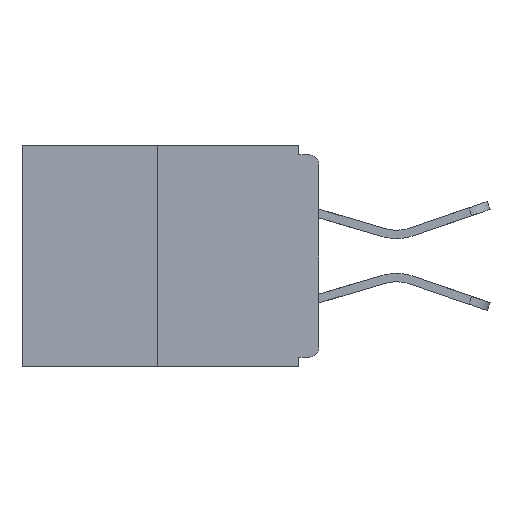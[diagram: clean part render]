
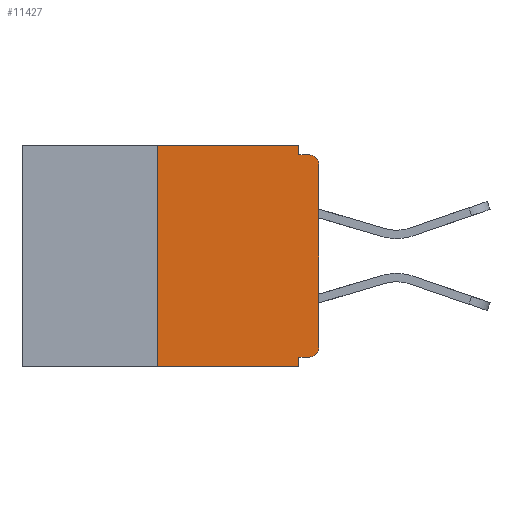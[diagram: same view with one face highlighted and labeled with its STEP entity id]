
A CAD part, left-side view. The second image highlights one B-rep face of the part: STEP entity #11427.
In plain terms, the highlighted planar face has unit normal (-1, 0, 0).
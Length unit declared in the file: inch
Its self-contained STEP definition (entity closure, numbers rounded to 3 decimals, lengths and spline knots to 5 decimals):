
#107 = VECTOR ( 'NONE', #7670, 39.37008 ) ;
#409 = VERTEX_POINT ( 'NONE', #15569 ) ;
#592 = CARTESIAN_POINT ( 'NONE',  ( 0., 0.031, -0.328 ) ) ;
#746 = DIRECTION ( 'NONE',  ( 0., -1., 0. ) ) ;
#1285 = CARTESIAN_POINT ( 'NONE',  ( 0., 0., -0.015 ) ) ;
#1551 = LINE ( 'NONE', #4420, #9061 ) ;
#1631 = FACE_OUTER_BOUND ( 'NONE', #15533, .T. ) ;
#1824 = VECTOR ( 'NONE', #6042, 39.37008 ) ;
#1983 = DIRECTION ( 'NONE',  ( 0., 0., -1. ) ) ;
#2029 = EDGE_CURVE ( 'NONE', #6592, #18800, #13222, .T. ) ;
#2368 = ORIENTED_EDGE ( 'NONE', *, *, #14541, .T. ) ;
#2516 = DIRECTION ( 'NONE',  ( -1., 0., 0. ) ) ;
#2606 = EDGE_CURVE ( 'NONE', #8097, #13336, #1551, .T. ) ;
#2752 = AXIS2_PLACEMENT_3D ( 'NONE', #11865, #2516, #14719 ) ;
#2773 = DIRECTION ( 'NONE',  ( 0., 0., 1. ) ) ;
#2797 = VERTEX_POINT ( 'NONE', #3875 ) ;
#2963 = CIRCLE ( 'NONE', #6672, 0.015 ) ;
#3875 = CARTESIAN_POINT ( 'NONE',  ( 0., 0.25, 0. ) ) ;
#4314 = ORIENTED_EDGE ( 'NONE', *, *, #12653, .F. ) ;
#4420 = CARTESIAN_POINT ( 'NONE',  ( 0., 0., -0.328 ) ) ;
#5596 = DIRECTION ( 'NONE',  ( 0., 0., -1. ) ) ;
#5668 = ORIENTED_EDGE ( 'NONE', *, *, #13982, .F. ) ;
#6042 = DIRECTION ( 'NONE',  ( 0., 0., -1. ) ) ;
#6216 = CIRCLE ( 'NONE', #2752, 0.015 ) ;
#6592 = VERTEX_POINT ( 'NONE', #8459 ) ;
#6672 = AXIS2_PLACEMENT_3D ( 'NONE', #15354, #16957, #12325 ) ;
#7051 = VECTOR ( 'NONE', #11698, 39.37008 ) ;
#7240 = EDGE_CURVE ( 'NONE', #9380, #2797, #7882, .T. ) ;
#7248 = ORIENTED_EDGE ( 'NONE', *, *, #12248, .T. ) ;
#7323 = LINE ( 'NONE', #1285, #10512 ) ;
#7670 = DIRECTION ( 'NONE',  ( 0., 0., 1. ) ) ;
#7882 = LINE ( 'NONE', #18591, #107 ) ;
#8097 = VERTEX_POINT ( 'NONE', #17648 ) ;
#8459 = CARTESIAN_POINT ( 'NONE',  ( 0., 0., -0.313 ) ) ;
#8615 = DIRECTION ( 'NONE',  ( 1., 0., 0. ) ) ;
#9061 = VECTOR ( 'NONE', #17041, 39.37008 ) ;
#9180 = EDGE_CURVE ( 'NONE', #2797, #10215, #15837, .T. ) ;
#9380 = VERTEX_POINT ( 'NONE', #18120 ) ;
#10215 = VERTEX_POINT ( 'NONE', #12199 ) ;
#10512 = VECTOR ( 'NONE', #12095, 39.37008 ) ;
#11166 = ORIENTED_EDGE ( 'NONE', *, *, #9180, .F. ) ;
#11296 = VERTEX_POINT ( 'NONE', #18190 ) ;
#11427 = ADVANCED_FACE ( 'NONE', ( #1631 ), #17907, .F. ) ;
#11698 = DIRECTION ( 'NONE',  ( 0., -1., 0. ) ) ;
#11805 = LINE ( 'NONE', #16374, #12565 ) ;
#11847 = AXIS2_PLACEMENT_3D ( 'NONE', #16366, #8615, #5596 ) ;
#11859 = CARTESIAN_POINT ( 'NONE',  ( 0., 0.031, 0. ) ) ;
#11865 = CARTESIAN_POINT ( 'NONE',  ( 0., 0.015, -0.313 ) ) ;
#11987 = EDGE_CURVE ( 'NONE', #9380, #409, #11805, .T. ) ;
#12095 = DIRECTION ( 'NONE',  ( 0., -1., 0. ) ) ;
#12199 = CARTESIAN_POINT ( 'NONE',  ( 0., 0.031, 0. ) ) ;
#12248 = EDGE_CURVE ( 'NONE', #8097, #6592, #6216, .T. ) ;
#12325 = DIRECTION ( 'NONE',  ( 0., 0., -1. ) ) ;
#12565 = VECTOR ( 'NONE', #746, 39.37008 ) ;
#12653 = EDGE_CURVE ( 'NONE', #13336, #409, #17656, .T. ) ;
#12885 = EDGE_CURVE ( 'NONE', #10215, #11296, #19572, .T. ) ;
#12974 = VECTOR ( 'NONE', #2773, 39.37008 ) ;
#13079 = ORIENTED_EDGE ( 'NONE', *, *, #11987, .T. ) ;
#13222 = LINE ( 'NONE', #15106, #12974 ) ;
#13336 = VERTEX_POINT ( 'NONE', #592 ) ;
#13982 = EDGE_CURVE ( 'NONE', #11296, #19750, #7323, .T. ) ;
#14348 = CARTESIAN_POINT ( 'NONE',  ( 0., 0., -0.03 ) ) ;
#14541 = EDGE_CURVE ( 'NONE', #18800, #19750, #2963, .T. ) ;
#14689 = VECTOR ( 'NONE', #1983, 39.37008 ) ;
#14719 = DIRECTION ( 'NONE',  ( 0., 0., -1. ) ) ;
#14742 = CARTESIAN_POINT ( 'NONE',  ( 0., 0.46, 0. ) ) ;
#15106 = CARTESIAN_POINT ( 'NONE',  ( 0., 0., 0. ) ) ;
#15354 = CARTESIAN_POINT ( 'NONE',  ( 0., 0.015, -0.03 ) ) ;
#15533 = EDGE_LOOP ( 'NONE', ( #11166, #19455, #13079, #4314, #17997, #7248, #18024, #2368, #5668, #16016 ) ) ;
#15569 = CARTESIAN_POINT ( 'NONE',  ( 0., 0.031, -0.343 ) ) ;
#15837 = LINE ( 'NONE', #14742, #7051 ) ;
#16016 = ORIENTED_EDGE ( 'NONE', *, *, #12885, .F. ) ;
#16279 = CARTESIAN_POINT ( 'NONE',  ( 0., 0.015, -0.015 ) ) ;
#16366 = CARTESIAN_POINT ( 'NONE',  ( 0., 0.46, 0. ) ) ;
#16374 = CARTESIAN_POINT ( 'NONE',  ( 0., 0.46, -0.343 ) ) ;
#16957 = DIRECTION ( 'NONE',  ( -1., 0., 0. ) ) ;
#17041 = DIRECTION ( 'NONE',  ( 0., 1., 0. ) ) ;
#17429 = CARTESIAN_POINT ( 'NONE',  ( 0., 0.031, -0.343 ) ) ;
#17648 = CARTESIAN_POINT ( 'NONE',  ( 0., 0.015, -0.328 ) ) ;
#17656 = LINE ( 'NONE', #17429, #14689 ) ;
#17907 = PLANE ( 'NONE',  #11847 ) ;
#17997 = ORIENTED_EDGE ( 'NONE', *, *, #2606, .F. ) ;
#18024 = ORIENTED_EDGE ( 'NONE', *, *, #2029, .T. ) ;
#18120 = CARTESIAN_POINT ( 'NONE',  ( 0., 0.25, -0.343 ) ) ;
#18190 = CARTESIAN_POINT ( 'NONE',  ( 0., 0.031, -0.015 ) ) ;
#18591 = CARTESIAN_POINT ( 'NONE',  ( 0., 0.25, 0. ) ) ;
#18800 = VERTEX_POINT ( 'NONE', #14348 ) ;
#19455 = ORIENTED_EDGE ( 'NONE', *, *, #7240, .F. ) ;
#19572 = LINE ( 'NONE', #11859, #1824 ) ;
#19750 = VERTEX_POINT ( 'NONE', #16279 ) ;
